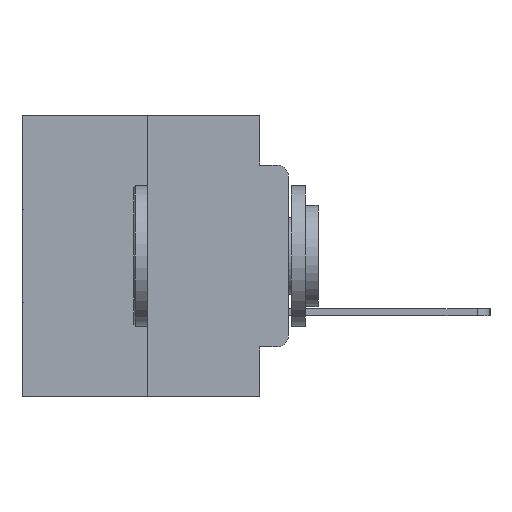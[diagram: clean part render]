
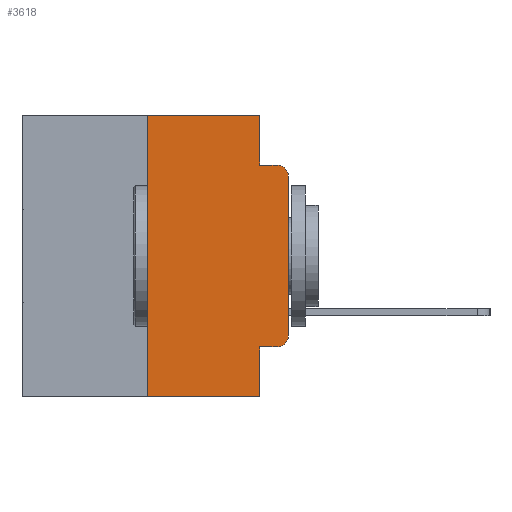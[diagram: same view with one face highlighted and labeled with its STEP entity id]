
A CAD part, left-side view. The second image highlights one B-rep face of the part: STEP entity #3618.
In plain terms, the highlighted planar face has unit normal (-1, 0, 0).
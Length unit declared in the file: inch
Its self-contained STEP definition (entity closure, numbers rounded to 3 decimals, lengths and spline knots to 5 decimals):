
#75 = VECTOR ( 'NONE', #21183, 39.37008 ) ;
#210 = EDGE_CURVE ( 'NONE', #711, #11040, #3805, .T. ) ;
#354 = DIRECTION ( 'NONE',  ( 0., -1., 0. ) ) ;
#711 = VERTEX_POINT ( 'NONE', #19298 ) ;
#956 = CARTESIAN_POINT ( 'NONE',  ( 0., 0.473, 0. ) ) ;
#1326 = DIRECTION ( 'NONE',  ( 1., 0., 0. ) ) ;
#1427 = DIRECTION ( 'NONE',  ( 0., 0., -1. ) ) ;
#1647 = VECTOR ( 'NONE', #15566, 39.37008 ) ;
#2189 = CARTESIAN_POINT ( 'NONE',  ( 0., 0.051, -0.0885 ) ) ;
#2417 = EDGE_CURVE ( 'NONE', #18092, #8997, #8730, .T. ) ;
#2667 = VECTOR ( 'NONE', #26046, 39.37008 ) ;
#3074 = CARTESIAN_POINT ( 'NONE',  ( 0., 0.473, -0.5 ) ) ;
#3166 = ORIENTED_EDGE ( 'NONE', *, *, #14010, .T. ) ;
#3557 = VECTOR ( 'NONE', #9035, 39.37008 ) ;
#3618 = ADVANCED_FACE ( 'NONE', ( #16189 ), #11715, .F. ) ;
#3805 = LINE ( 'NONE', #11538, #9083 ) ;
#4224 = AXIS2_PLACEMENT_3D ( 'NONE', #27928, #14879, #1427 ) ;
#5004 = EDGE_CURVE ( 'NONE', #19607, #27833, #15418, .T. ) ;
#6842 = VECTOR ( 'NONE', #27266, 39.37008 ) ;
#8730 = LINE ( 'NONE', #18315, #2667 ) ;
#8997 = VERTEX_POINT ( 'NONE', #10415 ) ;
#9035 = DIRECTION ( 'NONE',  ( 0., -1., 0. ) ) ;
#9083 = VECTOR ( 'NONE', #13816, 39.37008 ) ;
#9947 = CARTESIAN_POINT ( 'NONE',  ( 0., 0.051, -0.4115 ) ) ;
#9987 = DIRECTION ( 'NONE',  ( 0., 0., 1. ) ) ;
#10211 = ORIENTED_EDGE ( 'NONE', *, *, #14429, .T. ) ;
#10415 = CARTESIAN_POINT ( 'NONE',  ( 0., 0., -0.1085 ) ) ;
#10693 = CARTESIAN_POINT ( 'NONE',  ( 0., 0.051, -0.0885 ) ) ;
#10902 = ORIENTED_EDGE ( 'NONE', *, *, #24699, .F. ) ;
#11040 = VERTEX_POINT ( 'NONE', #10693 ) ;
#11223 = DIRECTION ( 'NONE',  ( -1., 0., 0. ) ) ;
#11264 = ORIENTED_EDGE ( 'NONE', *, *, #16251, .T. ) ;
#11538 = CARTESIAN_POINT ( 'NONE',  ( 0., 0.051, 0. ) ) ;
#11590 = ORIENTED_EDGE ( 'NONE', *, *, #19591, .F. ) ;
#11715 = PLANE ( 'NONE',  #23567 ) ;
#11855 = CARTESIAN_POINT ( 'NONE',  ( 0., 0.051, -0.5 ) ) ;
#13788 = CARTESIAN_POINT ( 'NONE',  ( 0., 0.25, 0. ) ) ;
#13816 = DIRECTION ( 'NONE',  ( 0., 0., -1. ) ) ;
#13924 = CARTESIAN_POINT ( 'NONE',  ( 0., 0.473, 0. ) ) ;
#14010 = EDGE_CURVE ( 'NONE', #19607, #23392, #24993, .T. ) ;
#14022 = CARTESIAN_POINT ( 'NONE',  ( 0., 0.25, -0.5 ) ) ;
#14042 = CIRCLE ( 'NONE', #4224, 0.02 ) ;
#14429 = EDGE_CURVE ( 'NONE', #8997, #18018, #25640, .T. ) ;
#14636 = VERTEX_POINT ( 'NONE', #22888 ) ;
#14742 = VECTOR ( 'NONE', #9987, 39.37008 ) ;
#14879 = DIRECTION ( 'NONE',  ( -1., 0., 0. ) ) ;
#15360 = LINE ( 'NONE', #24367, #3557 ) ;
#15418 = LINE ( 'NONE', #25714, #14742 ) ;
#15566 = DIRECTION ( 'NONE',  ( 0., -1., 0. ) ) ;
#16056 = AXIS2_PLACEMENT_3D ( 'NONE', #24346, #11223, #26494 ) ;
#16160 = EDGE_LOOP ( 'NONE', ( #26950, #10211, #10902, #22544, #11590, #24614, #3166, #26627, #11264, #28609 ) ) ;
#16189 = FACE_OUTER_BOUND ( 'NONE', #16160, .T. ) ;
#16251 = EDGE_CURVE ( 'NONE', #20328, #14636, #15360, .T. ) ;
#16786 = CARTESIAN_POINT ( 'NONE',  ( 0., 0.051, 0. ) ) ;
#16886 = LINE ( 'NONE', #13924, #22013 ) ;
#18018 = VERTEX_POINT ( 'NONE', #26337 ) ;
#18026 = LINE ( 'NONE', #16786, #75 ) ;
#18092 = VERTEX_POINT ( 'NONE', #19938 ) ;
#18315 = CARTESIAN_POINT ( 'NONE',  ( 0., 0., 0. ) ) ;
#19298 = CARTESIAN_POINT ( 'NONE',  ( 0., 0.051, 0. ) ) ;
#19591 = EDGE_CURVE ( 'NONE', #27833, #711, #16886, .T. ) ;
#19607 = VERTEX_POINT ( 'NONE', #14022 ) ;
#19938 = CARTESIAN_POINT ( 'NONE',  ( 0., 0., -0.3915 ) ) ;
#20328 = VERTEX_POINT ( 'NONE', #9947 ) ;
#21183 = DIRECTION ( 'NONE',  ( 0., 0., -1. ) ) ;
#22013 = VECTOR ( 'NONE', #354, 39.37008 ) ;
#22544 = ORIENTED_EDGE ( 'NONE', *, *, #210, .F. ) ;
#22888 = CARTESIAN_POINT ( 'NONE',  ( 0., 0.02, -0.4115 ) ) ;
#23392 = VERTEX_POINT ( 'NONE', #11855 ) ;
#23567 = AXIS2_PLACEMENT_3D ( 'NONE', #956, #1326, #28155 ) ;
#23613 = EDGE_CURVE ( 'NONE', #14636, #18092, #14042, .T. ) ;
#24346 = CARTESIAN_POINT ( 'NONE',  ( 0., 0.02, -0.1085 ) ) ;
#24367 = CARTESIAN_POINT ( 'NONE',  ( 0., 0.051, -0.4115 ) ) ;
#24614 = ORIENTED_EDGE ( 'NONE', *, *, #5004, .F. ) ;
#24699 = EDGE_CURVE ( 'NONE', #11040, #18018, #25275, .T. ) ;
#24993 = LINE ( 'NONE', #3074, #6842 ) ;
#25275 = LINE ( 'NONE', #2189, #1647 ) ;
#25614 = EDGE_CURVE ( 'NONE', #20328, #23392, #18026, .T. ) ;
#25640 = CIRCLE ( 'NONE', #16056, 0.02 ) ;
#25714 = CARTESIAN_POINT ( 'NONE',  ( 0., 0.25, 0. ) ) ;
#26046 = DIRECTION ( 'NONE',  ( 0., 0., 1. ) ) ;
#26337 = CARTESIAN_POINT ( 'NONE',  ( 0., 0.02, -0.0885 ) ) ;
#26494 = DIRECTION ( 'NONE',  ( 0., 0., -1. ) ) ;
#26627 = ORIENTED_EDGE ( 'NONE', *, *, #25614, .F. ) ;
#26950 = ORIENTED_EDGE ( 'NONE', *, *, #2417, .T. ) ;
#27266 = DIRECTION ( 'NONE',  ( 0., -1., 0. ) ) ;
#27833 = VERTEX_POINT ( 'NONE', #13788 ) ;
#27928 = CARTESIAN_POINT ( 'NONE',  ( 0., 0.02, -0.3915 ) ) ;
#28155 = DIRECTION ( 'NONE',  ( 0., 0., -1. ) ) ;
#28609 = ORIENTED_EDGE ( 'NONE', *, *, #23613, .T. ) ;
